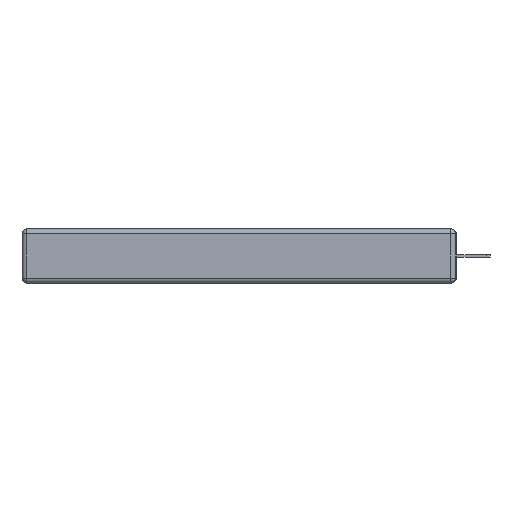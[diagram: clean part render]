
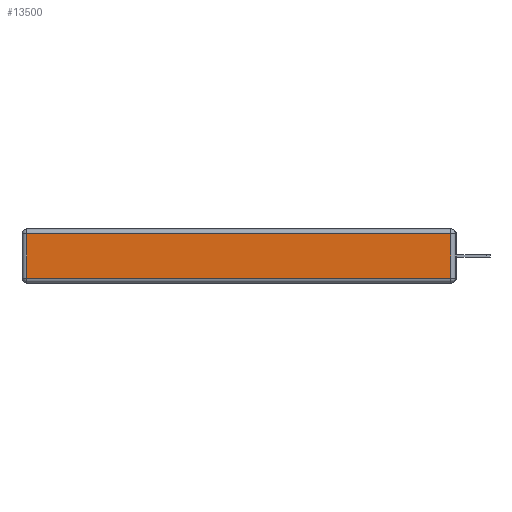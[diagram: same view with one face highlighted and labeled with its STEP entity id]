
A CAD part, left-side view. The second image highlights one B-rep face of the part: STEP entity #13500.
In plain terms, the highlighted planar face has unit normal (-1, 0, 0).
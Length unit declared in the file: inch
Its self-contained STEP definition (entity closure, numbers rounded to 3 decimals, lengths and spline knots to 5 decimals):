
#10 = LINE ( 'NONE', #15647, #1095 ) ;
#84 = ORIENTED_EDGE ( 'NONE', *, *, #15133, .T. ) ;
#214 = VERTEX_POINT ( 'NONE', #3803 ) ;
#1095 = VECTOR ( 'NONE', #8979, 39.37008 ) ;
#1627 = CARTESIAN_POINT ( 'NONE',  ( 0., 0., -0.343 ) ) ;
#2123 = VERTEX_POINT ( 'NONE', #10020 ) ;
#2350 = ORIENTED_EDGE ( 'NONE', *, *, #17502, .T. ) ;
#3803 = CARTESIAN_POINT ( 'NONE',  ( 0., 2.72, -0.03 ) ) ;
#3969 = CARTESIAN_POINT ( 'NONE',  ( 0., 2.72, -0.343 ) ) ;
#4190 = DIRECTION ( 'NONE',  ( 0., 0., 1. ) ) ;
#5151 = CARTESIAN_POINT ( 'NONE',  ( 0., 0.03, -0.313 ) ) ;
#5333 = DIRECTION ( 'NONE',  ( 0., 0., -1. ) ) ;
#5475 = AXIS2_PLACEMENT_3D ( 'NONE', #1627, #15298, #4190 ) ;
#5515 = PLANE ( 'NONE',  #5475 ) ;
#5572 = VECTOR ( 'NONE', #11994, 39.37008 ) ;
#6243 = EDGE_CURVE ( 'NONE', #12039, #9239, #17494, .T. ) ;
#7299 = DIRECTION ( 'NONE',  ( 0., -1., 0. ) ) ;
#8583 = LINE ( 'NONE', #13619, #5572 ) ;
#8979 = DIRECTION ( 'NONE',  ( 0., 1., 0. ) ) ;
#9125 = VECTOR ( 'NONE', #5333, 39.37008 ) ;
#9239 = VERTEX_POINT ( 'NONE', #5151 ) ;
#9970 = LINE ( 'NONE', #3969, #9125 ) ;
#10020 = CARTESIAN_POINT ( 'NONE',  ( 0., 0.03, -0.03 ) ) ;
#10391 = VECTOR ( 'NONE', #7299, 39.37008 ) ;
#11262 = ORIENTED_EDGE ( 'NONE', *, *, #17225, .T. ) ;
#11994 = DIRECTION ( 'NONE',  ( 0., 0., 1. ) ) ;
#12039 = VERTEX_POINT ( 'NONE', #14571 ) ;
#12556 = CARTESIAN_POINT ( 'NONE',  ( 0., 0., -0.313 ) ) ;
#12922 = ORIENTED_EDGE ( 'NONE', *, *, #6243, .T. ) ;
#13500 = ADVANCED_FACE ( 'NONE', ( #13746 ), #5515, .T. ) ;
#13619 = CARTESIAN_POINT ( 'NONE',  ( 0., 0.03, -0.343 ) ) ;
#13746 = FACE_OUTER_BOUND ( 'NONE', #17407, .T. ) ;
#14571 = CARTESIAN_POINT ( 'NONE',  ( 0., 2.72, -0.313 ) ) ;
#15133 = EDGE_CURVE ( 'NONE', #214, #12039, #9970, .T. ) ;
#15298 = DIRECTION ( 'NONE',  ( -1., 0., 0. ) ) ;
#15647 = CARTESIAN_POINT ( 'NONE',  ( 0., 2.75, -0.03 ) ) ;
#17225 = EDGE_CURVE ( 'NONE', #2123, #214, #10, .T. ) ;
#17407 = EDGE_LOOP ( 'NONE', ( #12922, #2350, #11262, #84 ) ) ;
#17494 = LINE ( 'NONE', #12556, #10391 ) ;
#17502 = EDGE_CURVE ( 'NONE', #9239, #2123, #8583, .T. ) ;
